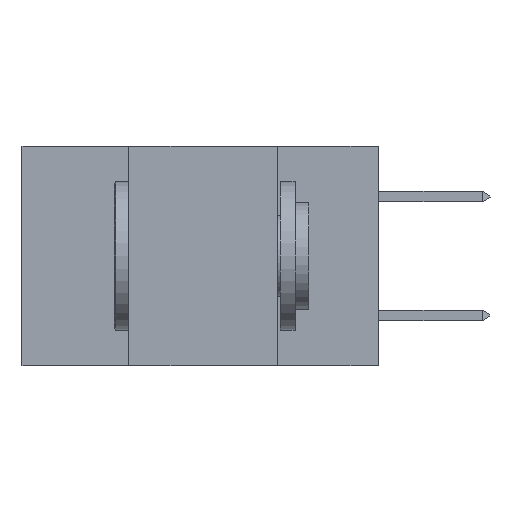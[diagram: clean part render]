
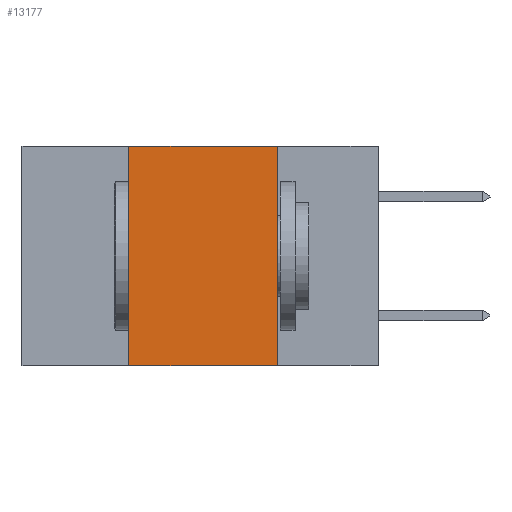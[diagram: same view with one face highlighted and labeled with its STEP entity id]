
A CAD part, left-side view. The second image highlights one B-rep face of the part: STEP entity #13177.
In plain terms, the highlighted planar face has unit normal (-1, 0, 0).
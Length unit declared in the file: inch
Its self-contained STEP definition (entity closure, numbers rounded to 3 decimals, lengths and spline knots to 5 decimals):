
#139 = ORIENTED_EDGE ( 'NONE', *, *, #14467, .F. ) ;
#1380 = CARTESIAN_POINT ( 'NONE',  ( 0., 0.6, -0.37 ) ) ;
#2950 = DIRECTION ( 'NONE',  ( 0., 0., -1. ) ) ;
#3007 = DIRECTION ( 'NONE',  ( 1., 0., 0. ) ) ;
#3412 = ORIENTED_EDGE ( 'NONE', *, *, #4768, .F. ) ;
#3889 = LINE ( 'NONE', #1380, #5762 ) ;
#3936 = ORIENTED_EDGE ( 'NONE', *, *, #5645, .T. ) ;
#4145 = LINE ( 'NONE', #12982, #9515 ) ;
#4429 = ORIENTED_EDGE ( 'NONE', *, *, #7888, .F. ) ;
#4484 = CARTESIAN_POINT ( 'NONE',  ( 0., 0.6, 0. ) ) ;
#4768 = EDGE_CURVE ( 'NONE', #16182, #17266, #4145, .T. ) ;
#5567 = AXIS2_PLACEMENT_3D ( 'NONE', #4484, #3007, #2950 ) ;
#5645 = EDGE_CURVE ( 'NONE', #13601, #13668, #3889, .T. ) ;
#5712 = PLANE ( 'NONE',  #5567 ) ;
#5738 = EDGE_LOOP ( 'NONE', ( #139, #3412, #4429, #3936 ) ) ;
#5762 = VECTOR ( 'NONE', #13317, 39.37008 ) ;
#6813 = CARTESIAN_POINT ( 'NONE',  ( 0., 0.17, -0.37 ) ) ;
#7547 = VECTOR ( 'NONE', #15349, 39.37008 ) ;
#7888 = EDGE_CURVE ( 'NONE', #13601, #16182, #11927, .T. ) ;
#7963 = CARTESIAN_POINT ( 'NONE',  ( 0., 0.42, 0. ) ) ;
#9515 = VECTOR ( 'NONE', #10215, 39.37008 ) ;
#9724 = CARTESIAN_POINT ( 'NONE',  ( 0., 0.17, 0. ) ) ;
#10000 = CARTESIAN_POINT ( 'NONE',  ( 0., 0.42, 0. ) ) ;
#10215 = DIRECTION ( 'NONE',  ( 0., -1., 0. ) ) ;
#11074 = DIRECTION ( 'NONE',  ( 0., 0., -1. ) ) ;
#11197 = CARTESIAN_POINT ( 'NONE',  ( 0., 0.17, 0. ) ) ;
#11590 = LINE ( 'NONE', #11197, #15810 ) ;
#11927 = LINE ( 'NONE', #10000, #7547 ) ;
#12982 = CARTESIAN_POINT ( 'NONE',  ( 0., 0.6, 0. ) ) ;
#13177 = ADVANCED_FACE ( 'NONE', ( #13754 ), #5712, .F. ) ;
#13317 = DIRECTION ( 'NONE',  ( 0., -1., 0. ) ) ;
#13368 = CARTESIAN_POINT ( 'NONE',  ( 0., 0.42, -0.37 ) ) ;
#13601 = VERTEX_POINT ( 'NONE', #13368 ) ;
#13668 = VERTEX_POINT ( 'NONE', #6813 ) ;
#13754 = FACE_OUTER_BOUND ( 'NONE', #5738, .T. ) ;
#14467 = EDGE_CURVE ( 'NONE', #17266, #13668, #11590, .T. ) ;
#15349 = DIRECTION ( 'NONE',  ( 0., 0., 1. ) ) ;
#15810 = VECTOR ( 'NONE', #11074, 39.37008 ) ;
#16182 = VERTEX_POINT ( 'NONE', #7963 ) ;
#17266 = VERTEX_POINT ( 'NONE', #9724 ) ;
